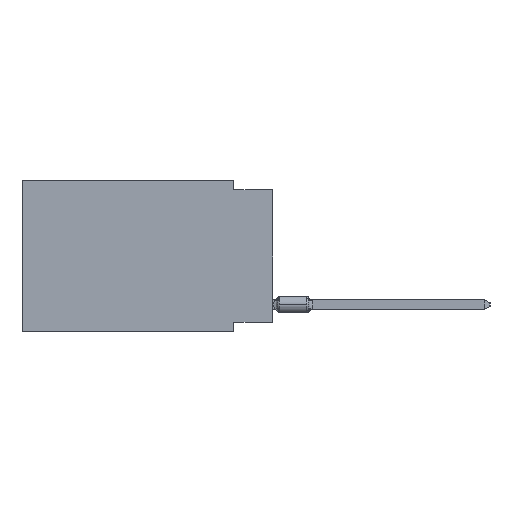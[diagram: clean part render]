
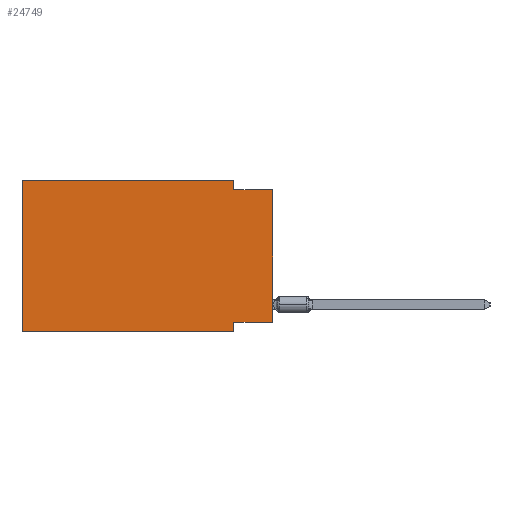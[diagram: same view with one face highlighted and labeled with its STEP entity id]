
A CAD part, left-side view. The second image highlights one B-rep face of the part: STEP entity #24749.
In plain terms, the highlighted planar face has unit normal (-1, 0, 0).
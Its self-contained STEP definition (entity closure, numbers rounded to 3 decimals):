
#294 = CARTESIAN_POINT ( 'NONE',  ( 0., 2.54, -9.906 ) ) ;
#3354 = CARTESIAN_POINT ( 'NONE',  ( 0., 16.383, 0. ) ) ;
#4126 = ORIENTED_EDGE ( 'NONE', *, *, #12659, .T. ) ;
#8409 = EDGE_CURVE ( 'NONE', #69099, #72354, #17481, .T. ) ;
#8790 = CARTESIAN_POINT ( 'NONE',  ( 0., 0., 0. ) ) ;
#9860 = DIRECTION ( 'NONE',  ( 0., 0., 1. ) ) ;
#10233 = EDGE_CURVE ( 'NONE', #38068, #69099, #61429, .T. ) ;
#10370 = EDGE_LOOP ( 'NONE', ( #42314, #48130, #13543, #20486, #40334, #4126, #49605, #35781 ) ) ;
#10539 = VERTEX_POINT ( 'NONE', #13101 ) ;
#10675 = AXIS2_PLACEMENT_3D ( 'NONE', #39799, #22159, #68161 ) ;
#11055 = DIRECTION ( 'NONE',  ( 0., -1., 0. ) ) ;
#12659 = EDGE_CURVE ( 'NONE', #44373, #32313, #59419, .T. ) ;
#13101 = CARTESIAN_POINT ( 'NONE',  ( 0., 0., -9.271 ) ) ;
#13543 = ORIENTED_EDGE ( 'NONE', *, *, #8409, .F. ) ;
#17481 = LINE ( 'NONE', #40876, #21252 ) ;
#18563 = EDGE_CURVE ( 'NONE', #44373, #38068, #56621, .T. ) ;
#18583 = CARTESIAN_POINT ( 'NONE',  ( 0., 0., -9.271 ) ) ;
#19641 = VECTOR ( 'NONE', #50186, 1000. ) ;
#20486 = ORIENTED_EDGE ( 'NONE', *, *, #10233, .F. ) ;
#20895 = EDGE_CURVE ( 'NONE', #36939, #32313, #56689, .T. ) ;
#21252 = VECTOR ( 'NONE', #64242, 1000. ) ;
#22159 = DIRECTION ( 'NONE',  ( 1., 0., 0. ) ) ;
#24749 = ADVANCED_FACE ( 'NONE', ( #40174 ), #27915, .F. ) ;
#25985 = EDGE_CURVE ( 'NONE', #72354, #68612, #27923, .T. ) ;
#27546 = CARTESIAN_POINT ( 'NONE',  ( 0., 2.54, -9.906 ) ) ;
#27698 = DIRECTION ( 'NONE',  ( 0., -1., 0. ) ) ;
#27915 = PLANE ( 'NONE',  #10675 ) ;
#27923 = LINE ( 'NONE', #51331, #35239 ) ;
#30279 = VECTOR ( 'NONE', #65914, 1000. ) ;
#31213 = CARTESIAN_POINT ( 'NONE',  ( 0., 2.54, 0. ) ) ;
#32313 = VERTEX_POINT ( 'NONE', #294 ) ;
#32810 = EDGE_CURVE ( 'NONE', #10539, #36939, #60728, .T. ) ;
#33794 = EDGE_CURVE ( 'NONE', #10539, #68612, #39053, .T. ) ;
#35239 = VECTOR ( 'NONE', #11055, 1000. ) ;
#35781 = ORIENTED_EDGE ( 'NONE', *, *, #32810, .F. ) ;
#36671 = VECTOR ( 'NONE', #66846, 1000. ) ;
#36939 = VERTEX_POINT ( 'NONE', #45175 ) ;
#38068 = VERTEX_POINT ( 'NONE', #42534 ) ;
#39053 = LINE ( 'NONE', #8790, #19641 ) ;
#39799 = CARTESIAN_POINT ( 'NONE',  ( 0., 16.383, 0. ) ) ;
#40174 = FACE_OUTER_BOUND ( 'NONE', #10370, .T. ) ;
#40334 = ORIENTED_EDGE ( 'NONE', *, *, #18563, .F. ) ;
#40876 = CARTESIAN_POINT ( 'NONE',  ( 0., 2.54, 0. ) ) ;
#42272 = VECTOR ( 'NONE', #27698, 1000. ) ;
#42314 = ORIENTED_EDGE ( 'NONE', *, *, #33794, .T. ) ;
#42534 = CARTESIAN_POINT ( 'NONE',  ( 0., 16.383, 0. ) ) ;
#44373 = VERTEX_POINT ( 'NONE', #48359 ) ;
#45175 = CARTESIAN_POINT ( 'NONE',  ( 0., 2.54, -9.271 ) ) ;
#48130 = ORIENTED_EDGE ( 'NONE', *, *, #25985, .F. ) ;
#48359 = CARTESIAN_POINT ( 'NONE',  ( 0., 16.383, -9.906 ) ) ;
#49605 = ORIENTED_EDGE ( 'NONE', *, *, #20895, .F. ) ;
#50186 = DIRECTION ( 'NONE',  ( 0., 0., 1. ) ) ;
#50954 = DIRECTION ( 'NONE',  ( 0., 0., -1. ) ) ;
#51331 = CARTESIAN_POINT ( 'NONE',  ( 0., 0., -0.635 ) ) ;
#56621 = LINE ( 'NONE', #3354, #66483 ) ;
#56689 = LINE ( 'NONE', #27546, #60458 ) ;
#59419 = LINE ( 'NONE', #66664, #30279 ) ;
#60458 = VECTOR ( 'NONE', #50954, 1000. ) ;
#60728 = LINE ( 'NONE', #18583, #36671 ) ;
#61429 = LINE ( 'NONE', #73318, #42272 ) ;
#61945 = CARTESIAN_POINT ( 'NONE',  ( 0., 2.54, -0.635 ) ) ;
#64242 = DIRECTION ( 'NONE',  ( 0., 0., -1. ) ) ;
#65914 = DIRECTION ( 'NONE',  ( 0., -1., 0. ) ) ;
#66180 = CARTESIAN_POINT ( 'NONE',  ( 0., 0., -0.635 ) ) ;
#66483 = VECTOR ( 'NONE', #9860, 1000. ) ;
#66664 = CARTESIAN_POINT ( 'NONE',  ( 0., 16.383, -9.906 ) ) ;
#66846 = DIRECTION ( 'NONE',  ( 0., 1., 0. ) ) ;
#68161 = DIRECTION ( 'NONE',  ( 0., 0., -1. ) ) ;
#68612 = VERTEX_POINT ( 'NONE', #66180 ) ;
#69099 = VERTEX_POINT ( 'NONE', #31213 ) ;
#72354 = VERTEX_POINT ( 'NONE', #61945 ) ;
#73318 = CARTESIAN_POINT ( 'NONE',  ( 0., 16.383, 0. ) ) ;
